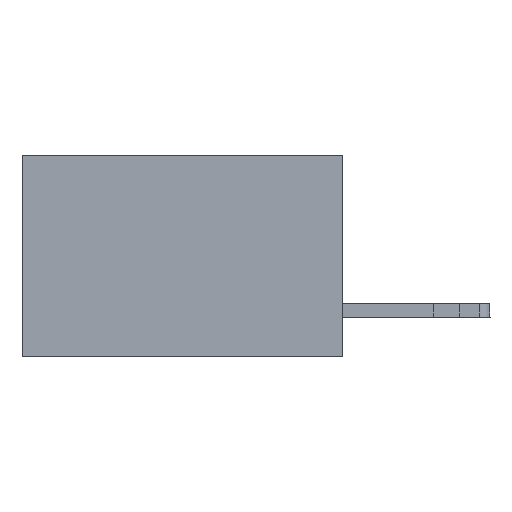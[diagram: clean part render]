
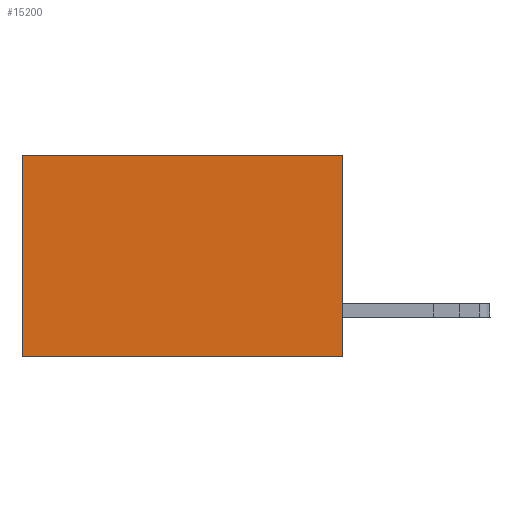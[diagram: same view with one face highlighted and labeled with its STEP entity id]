
A CAD part, left-side view. The second image highlights one B-rep face of the part: STEP entity #15200.
In plain terms, the highlighted planar face has unit normal (-1, 0, 0).
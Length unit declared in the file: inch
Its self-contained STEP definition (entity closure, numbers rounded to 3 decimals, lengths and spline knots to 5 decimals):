
#197 = AXIS2_PLACEMENT_3D ( 'NONE', #6889, #5583, #14694 ) ;
#663 = VERTEX_POINT ( 'NONE', #1452 ) ;
#760 = ORIENTED_EDGE ( 'NONE', *, *, #8173, .F. ) ;
#1191 = ORIENTED_EDGE ( 'NONE', *, *, #4693, .T. ) ;
#1452 = CARTESIAN_POINT ( 'NONE',  ( 0.277, 0.59, 0. ) ) ;
#2077 = CARTESIAN_POINT ( 'NONE',  ( 0.277, 0.59, -0.37 ) ) ;
#2462 = CARTESIAN_POINT ( 'NONE',  ( 0.277, 0., -0.37 ) ) ;
#2473 = LINE ( 'NONE', #2077, #5580 ) ;
#3100 = LINE ( 'NONE', #13974, #13965 ) ;
#3162 = CARTESIAN_POINT ( 'NONE',  ( 0.277, 0., -0.37 ) ) ;
#4382 = EDGE_LOOP ( 'NONE', ( #7511, #11373, #760, #1191 ) ) ;
#4563 = DIRECTION ( 'NONE',  ( 0., 0., -1. ) ) ;
#4621 = DIRECTION ( 'NONE',  ( 0., 1., 0. ) ) ;
#4693 = EDGE_CURVE ( 'NONE', #11384, #663, #3100, .T. ) ;
#4761 = FACE_OUTER_BOUND ( 'NONE', #4382, .T. ) ;
#4792 = CARTESIAN_POINT ( 'NONE',  ( 0.277, 0., 0. ) ) ;
#5101 = VERTEX_POINT ( 'NONE', #9725 ) ;
#5580 = VECTOR ( 'NONE', #4563, 39.37008 ) ;
#5583 = DIRECTION ( 'NONE',  ( 1., 0., 0. ) ) ;
#6809 = VERTEX_POINT ( 'NONE', #2462 ) ;
#6889 = CARTESIAN_POINT ( 'NONE',  ( 0.277, 0., -0.37 ) ) ;
#7418 = DIRECTION ( 'NONE',  ( 0., 1., 0. ) ) ;
#7511 = ORIENTED_EDGE ( 'NONE', *, *, #8961, .T. ) ;
#8173 = EDGE_CURVE ( 'NONE', #11384, #6809, #14390, .T. ) ;
#8479 = DIRECTION ( 'NONE',  ( 0., 0., -1. ) ) ;
#8961 = EDGE_CURVE ( 'NONE', #663, #5101, #2473, .T. ) ;
#9725 = CARTESIAN_POINT ( 'NONE',  ( 0.277, 0.59, -0.37 ) ) ;
#10799 = EDGE_CURVE ( 'NONE', #6809, #5101, #13887, .T. ) ;
#11230 = CARTESIAN_POINT ( 'NONE',  ( 0.277, 0., -0.37 ) ) ;
#11373 = ORIENTED_EDGE ( 'NONE', *, *, #10799, .F. ) ;
#11384 = VERTEX_POINT ( 'NONE', #4792 ) ;
#11387 = VECTOR ( 'NONE', #8479, 39.37008 ) ;
#13420 = PLANE ( 'NONE',  #197 ) ;
#13499 = VECTOR ( 'NONE', #4621, 39.37008 ) ;
#13887 = LINE ( 'NONE', #11230, #13499 ) ;
#13965 = VECTOR ( 'NONE', #7418, 39.37008 ) ;
#13974 = CARTESIAN_POINT ( 'NONE',  ( 0.277, 0., 0. ) ) ;
#14390 = LINE ( 'NONE', #3162, #11387 ) ;
#14694 = DIRECTION ( 'NONE',  ( 0., 0., -1. ) ) ;
#15200 = ADVANCED_FACE ( 'NONE', ( #4761 ), #13420, .F. ) ;
